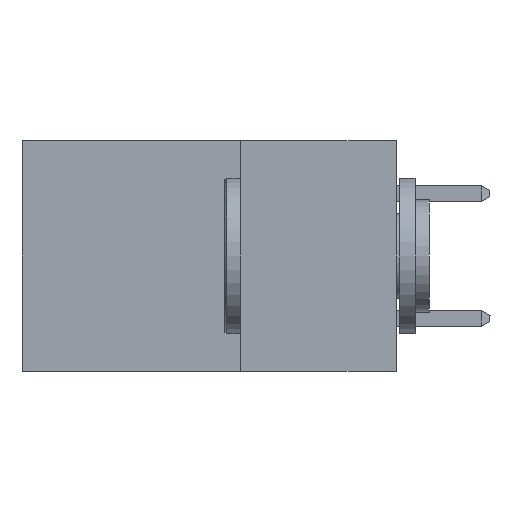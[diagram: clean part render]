
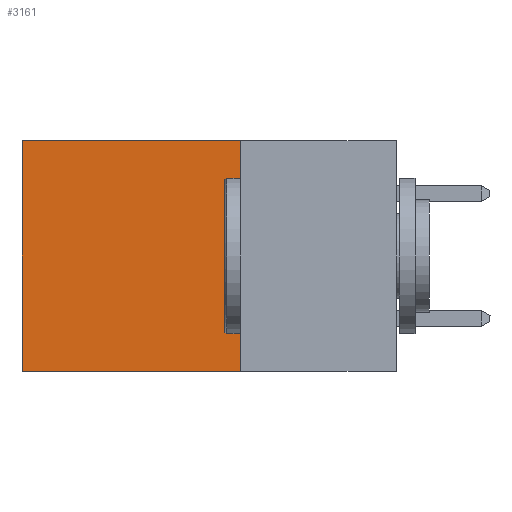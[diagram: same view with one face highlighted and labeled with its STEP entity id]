
A CAD part, left-side view. The second image highlights one B-rep face of the part: STEP entity #3161.
In plain terms, the highlighted planar face has unit normal (-1, 0, 0).
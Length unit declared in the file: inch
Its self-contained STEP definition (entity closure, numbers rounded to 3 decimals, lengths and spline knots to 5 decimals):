
#1387 = LINE ( 'NONE', #25148, #5241 ) ;
#1394 = VERTEX_POINT ( 'NONE', #3298 ) ;
#3161 = ADVANCED_FACE ( 'NONE', ( #19680 ), #7245, .F. ) ;
#3298 = CARTESIAN_POINT ( 'NONE',  ( 0.298, 0.25, -0.37 ) ) ;
#4748 = DIRECTION ( 'NONE',  ( 0., 1., 0. ) ) ;
#5030 = VERTEX_POINT ( 'NONE', #20709 ) ;
#5160 = CARTESIAN_POINT ( 'NONE',  ( 0.298, 0.25, 0. ) ) ;
#5241 = VECTOR ( 'NONE', #4748, 39.37008 ) ;
#5878 = VECTOR ( 'NONE', #19745, 39.37008 ) ;
#6028 = ORIENTED_EDGE ( 'NONE', *, *, #28339, .T. ) ;
#7022 = CARTESIAN_POINT ( 'NONE',  ( 0.298, 0.6, 0. ) ) ;
#7245 = PLANE ( 'NONE',  #27776 ) ;
#9021 = EDGE_LOOP ( 'NONE', ( #6028, #25499, #18111, #12198 ) ) ;
#9228 = VECTOR ( 'NONE', #25909, 39.37008 ) ;
#9680 = CARTESIAN_POINT ( 'NONE',  ( 0.298, 0.25, -0.37 ) ) ;
#11919 = LINE ( 'NONE', #22292, #5878 ) ;
#12023 = DIRECTION ( 'NONE',  ( 1., 0., 0. ) ) ;
#12078 = LINE ( 'NONE', #16942, #9228 ) ;
#12198 = ORIENTED_EDGE ( 'NONE', *, *, #13432, .T. ) ;
#13432 = EDGE_CURVE ( 'NONE', #5030, #21845, #1387, .T. ) ;
#16942 = CARTESIAN_POINT ( 'NONE',  ( 0.298, 0.25, 0. ) ) ;
#18011 = VECTOR ( 'NONE', #28027, 39.37008 ) ;
#18111 = ORIENTED_EDGE ( 'NONE', *, *, #18309, .F. ) ;
#18309 = EDGE_CURVE ( 'NONE', #5030, #1394, #12078, .T. ) ;
#18867 = DIRECTION ( 'NONE',  ( 0., 0., -1. ) ) ;
#19680 = FACE_OUTER_BOUND ( 'NONE', #9021, .T. ) ;
#19745 = DIRECTION ( 'NONE',  ( 0., 0., -1. ) ) ;
#19888 = EDGE_CURVE ( 'NONE', #1394, #20701, #20477, .T. ) ;
#20477 = LINE ( 'NONE', #9680, #18011 ) ;
#20701 = VERTEX_POINT ( 'NONE', #25471 ) ;
#20709 = CARTESIAN_POINT ( 'NONE',  ( 0.298, 0.25, 0. ) ) ;
#21845 = VERTEX_POINT ( 'NONE', #7022 ) ;
#22292 = CARTESIAN_POINT ( 'NONE',  ( 0.298, 0.6, 0. ) ) ;
#25148 = CARTESIAN_POINT ( 'NONE',  ( 0.298, 0.25, 0. ) ) ;
#25471 = CARTESIAN_POINT ( 'NONE',  ( 0.298, 0.6, -0.37 ) ) ;
#25499 = ORIENTED_EDGE ( 'NONE', *, *, #19888, .F. ) ;
#25909 = DIRECTION ( 'NONE',  ( 0., 0., -1. ) ) ;
#27776 = AXIS2_PLACEMENT_3D ( 'NONE', #5160, #12023, #18867 ) ;
#28027 = DIRECTION ( 'NONE',  ( 0., 1., 0. ) ) ;
#28339 = EDGE_CURVE ( 'NONE', #21845, #20701, #11919, .T. ) ;
